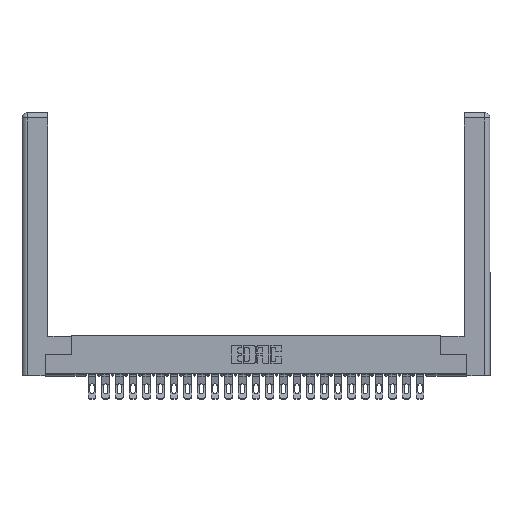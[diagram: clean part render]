
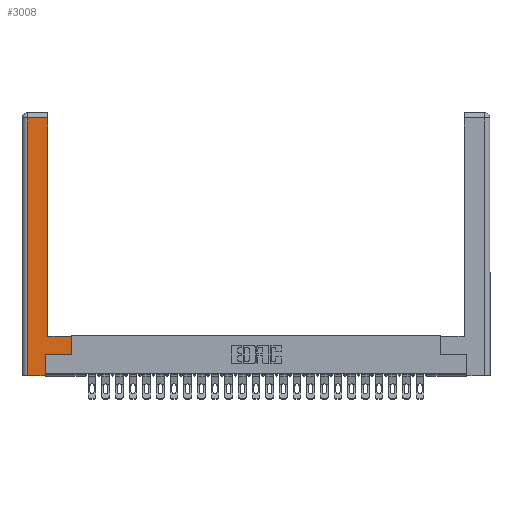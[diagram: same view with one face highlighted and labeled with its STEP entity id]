
A CAD part, top view. The second image highlights one B-rep face of the part: STEP entity #3008.
In plain terms, the highlighted planar face has unit normal (0, 0, 1).
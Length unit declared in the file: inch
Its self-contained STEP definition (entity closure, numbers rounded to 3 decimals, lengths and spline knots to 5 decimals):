
#813 = PLANE ( 'NONE',  #3374 ) ;
#2536 = VECTOR ( 'NONE', #16040, 39.37008 ) ;
#2538 = ORIENTED_EDGE ( 'NONE', *, *, #20200, .T. ) ;
#2550 = DIRECTION ( 'NONE',  ( 0., -1., 0. ) ) ;
#3004 = EDGE_CURVE ( 'NONE', #15706, #27694, #23919, .T. ) ;
#3008 = ADVANCED_FACE ( 'NONE', ( #27471 ), #813, .F. ) ;
#3068 = CARTESIAN_POINT ( 'NONE',  ( 0.265, 0., 0. ) ) ;
#3336 = DIRECTION ( 'NONE',  ( 0., 0., -1. ) ) ;
#3374 = AXIS2_PLACEMENT_3D ( 'NONE', #18271, #3336, #23292 ) ;
#3554 = CARTESIAN_POINT ( 'NONE',  ( 0.0615, 2.94, 0. ) ) ;
#4229 = ORIENTED_EDGE ( 'NONE', *, *, #18446, .T. ) ;
#4385 = VECTOR ( 'NONE', #31108, 39.37008 ) ;
#4626 = CARTESIAN_POINT ( 'NONE',  ( 0.265, 0.245, 0. ) ) ;
#4750 = VECTOR ( 'NONE', #18010, 39.37008 ) ;
#4783 = LINE ( 'NONE', #4626, #30225 ) ;
#6168 = ORIENTED_EDGE ( 'NONE', *, *, #29495, .T. ) ;
#6497 = LINE ( 'NONE', #19691, #22141 ) ;
#7534 = CARTESIAN_POINT ( 'NONE',  ( 0.265, 0., 0. ) ) ;
#7612 = VECTOR ( 'NONE', #13869, 39.37008 ) ;
#7911 = VERTEX_POINT ( 'NONE', #11641 ) ;
#8007 = LINE ( 'NONE', #10577, #2536 ) ;
#8210 = EDGE_CURVE ( 'NONE', #29172, #25132, #20940, .T. ) ;
#9758 = EDGE_CURVE ( 'NONE', #27694, #20152, #6497, .T. ) ;
#10181 = EDGE_CURVE ( 'NONE', #25132, #7911, #26845, .T. ) ;
#10218 = CARTESIAN_POINT ( 'NONE',  ( 0.565, 0.245, 0. ) ) ;
#10443 = DIRECTION ( 'NONE',  ( 0., 1., 0. ) ) ;
#10577 = CARTESIAN_POINT ( 'NONE',  ( 0.295, 0.45, 0. ) ) ;
#11641 = CARTESIAN_POINT ( 'NONE',  ( 0.565, 0.45, 0. ) ) ;
#12121 = DIRECTION ( 'NONE',  ( 0., 1., 0. ) ) ;
#12184 = EDGE_LOOP ( 'NONE', ( #2538, #25395, #26487, #30849, #6168, #14817, #23865, #4229 ) ) ;
#13869 = DIRECTION ( 'NONE',  ( 1., 0., 0. ) ) ;
#14108 = LINE ( 'NONE', #28226, #4750 ) ;
#14817 = ORIENTED_EDGE ( 'NONE', *, *, #8210, .T. ) ;
#14892 = DIRECTION ( 'NONE',  ( 1., 0., 0. ) ) ;
#15032 = CARTESIAN_POINT ( 'NONE',  ( 0.0615, 2.94, 0. ) ) ;
#15706 = VERTEX_POINT ( 'NONE', #24317 ) ;
#16040 = DIRECTION ( 'NONE',  ( -1., 0., 0. ) ) ;
#17026 = VERTEX_POINT ( 'NONE', #3068 ) ;
#18010 = DIRECTION ( 'NONE',  ( 0., 1., 0. ) ) ;
#18271 = CARTESIAN_POINT ( 'NONE',  ( 0., 0., 0. ) ) ;
#18446 = EDGE_CURVE ( 'NONE', #7911, #18633, #8007, .T. ) ;
#18633 = VERTEX_POINT ( 'NONE', #18675 ) ;
#18675 = CARTESIAN_POINT ( 'NONE',  ( 0.295, 0.45, 0. ) ) ;
#18968 = CARTESIAN_POINT ( 'NONE',  ( 0.265, 0.245, 0. ) ) ;
#19691 = CARTESIAN_POINT ( 'NONE',  ( 0.0615, 0., 0. ) ) ;
#20152 = VERTEX_POINT ( 'NONE', #22953 ) ;
#20200 = EDGE_CURVE ( 'NONE', #18633, #15706, #14108, .T. ) ;
#20940 = LINE ( 'NONE', #10218, #7612 ) ;
#20961 = VECTOR ( 'NONE', #14892, 39.37008 ) ;
#22141 = VECTOR ( 'NONE', #2550, 39.37008 ) ;
#22953 = CARTESIAN_POINT ( 'NONE',  ( 0.0615, 0., 0. ) ) ;
#23292 = DIRECTION ( 'NONE',  ( -1., 0., 0. ) ) ;
#23865 = ORIENTED_EDGE ( 'NONE', *, *, #10181, .T. ) ;
#23919 = LINE ( 'NONE', #3554, #4385 ) ;
#24317 = CARTESIAN_POINT ( 'NONE',  ( 0.295, 2.94, 0. ) ) ;
#24894 = LINE ( 'NONE', #7534, #20961 ) ;
#25132 = VERTEX_POINT ( 'NONE', #27898 ) ;
#25395 = ORIENTED_EDGE ( 'NONE', *, *, #3004, .T. ) ;
#26487 = ORIENTED_EDGE ( 'NONE', *, *, #9758, .T. ) ;
#26845 = LINE ( 'NONE', #30610, #30357 ) ;
#27161 = EDGE_CURVE ( 'NONE', #20152, #17026, #24894, .T. ) ;
#27471 = FACE_OUTER_BOUND ( 'NONE', #12184, .T. ) ;
#27694 = VERTEX_POINT ( 'NONE', #15032 ) ;
#27898 = CARTESIAN_POINT ( 'NONE',  ( 0.565, 0.245, 0. ) ) ;
#28226 = CARTESIAN_POINT ( 'NONE',  ( 0.295, 3., 0. ) ) ;
#29172 = VERTEX_POINT ( 'NONE', #18968 ) ;
#29495 = EDGE_CURVE ( 'NONE', #17026, #29172, #4783, .T. ) ;
#30225 = VECTOR ( 'NONE', #12121, 39.37008 ) ;
#30357 = VECTOR ( 'NONE', #10443, 39.37008 ) ;
#30610 = CARTESIAN_POINT ( 'NONE',  ( 0.565, 0.45, 0. ) ) ;
#30849 = ORIENTED_EDGE ( 'NONE', *, *, #27161, .T. ) ;
#31108 = DIRECTION ( 'NONE',  ( -1., 0., 0. ) ) ;
